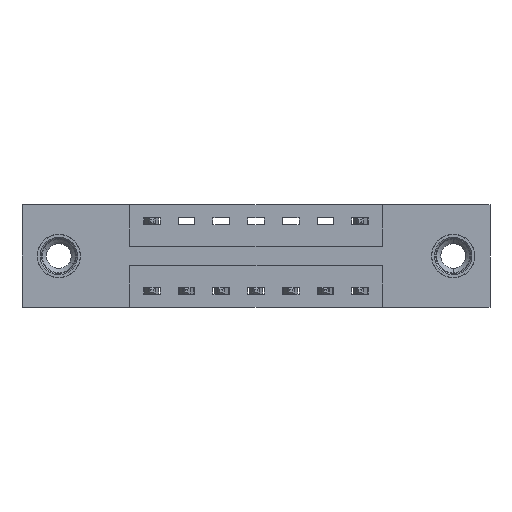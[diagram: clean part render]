
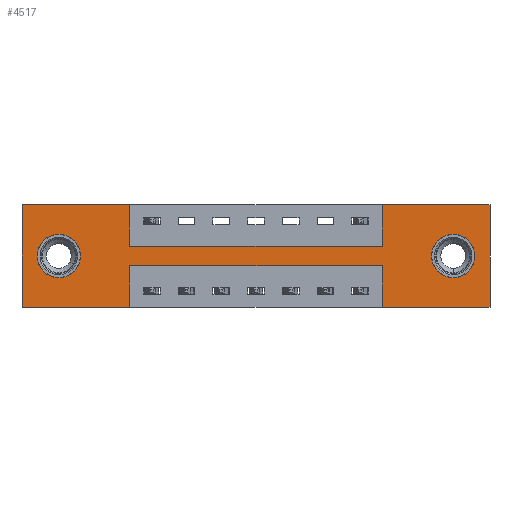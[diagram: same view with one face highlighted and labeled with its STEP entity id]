
A CAD part, front view. The second image highlights one B-rep face of the part: STEP entity #4517.
In plain terms, the highlighted planar face has unit normal (0, -1, 0).
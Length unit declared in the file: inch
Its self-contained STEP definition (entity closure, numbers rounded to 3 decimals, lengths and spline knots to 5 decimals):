
#27 = LINE ( 'NONE', #3414, #8600 ) ;
#93 = CARTESIAN_POINT ( 'NONE',  ( 1.2975, 0., -0.37 ) ) ;
#106 = CARTESIAN_POINT ( 'NONE',  ( 0.3875, 0., 0. ) ) ;
#147 = ORIENTED_EDGE ( 'NONE', *, *, #5257, .T. ) ;
#164 = VERTEX_POINT ( 'NONE', #93 ) ;
#167 = EDGE_CURVE ( 'NONE', #8975, #1400, #3425, .T. ) ;
#195 = CIRCLE ( 'NONE', #6165, 0.078 ) ;
#241 = CARTESIAN_POINT ( 'NONE',  ( 0.1325, 0., -0.263 ) ) ;
#291 = CARTESIAN_POINT ( 'NONE',  ( 0., 0., 0. ) ) ;
#565 = CARTESIAN_POINT ( 'NONE',  ( 0.1325, 0., -0.185 ) ) ;
#638 = CARTESIAN_POINT ( 'NONE',  ( 1.5525, 0., -0.263 ) ) ;
#639 = FACE_OUTER_BOUND ( 'NONE', #1988, .T. ) ;
#648 = AXIS2_PLACEMENT_3D ( 'NONE', #3900, #9489, #4722 ) ;
#661 = VECTOR ( 'NONE', #890, 39.37008 ) ;
#701 = CARTESIAN_POINT ( 'NONE',  ( 0., 0., -0.37 ) ) ;
#730 = VERTEX_POINT ( 'NONE', #6045 ) ;
#732 = EDGE_CURVE ( 'NONE', #3768, #1981, #9883, .T. ) ;
#786 = EDGE_CURVE ( 'NONE', #5219, #9329, #1160, .T. ) ;
#890 = DIRECTION ( 'NONE',  ( 0., 0., -1. ) ) ;
#899 = VECTOR ( 'NONE', #8381, 39.37008 ) ;
#1026 = DIRECTION ( 'NONE',  ( 0., 1., 0. ) ) ;
#1062 = ORIENTED_EDGE ( 'NONE', *, *, #4752, .F. ) ;
#1160 = LINE ( 'NONE', #1279, #899 ) ;
#1279 = CARTESIAN_POINT ( 'NONE',  ( 1.2975, 0., 0. ) ) ;
#1289 = LINE ( 'NONE', #8566, #7407 ) ;
#1358 = EDGE_CURVE ( 'NONE', #6492, #10025, #4766, .T. ) ;
#1366 = EDGE_LOOP ( 'NONE', ( #147, #7318 ) ) ;
#1400 = VERTEX_POINT ( 'NONE', #241 ) ;
#1449 = VERTEX_POINT ( 'NONE', #9149 ) ;
#1770 = VECTOR ( 'NONE', #5066, 39.37008 ) ;
#1893 = EDGE_CURVE ( 'NONE', #10025, #5219, #9355, .T. ) ;
#1908 = CIRCLE ( 'NONE', #6299, 0.078 ) ;
#1981 = VERTEX_POINT ( 'NONE', #8989 ) ;
#1988 = EDGE_LOOP ( 'NONE', ( #5203, #6474, #5142, #5419, #5060, #6479, #5100, #6022, #7809, #1062, #4306, #5007 ) ) ;
#2001 = VERTEX_POINT ( 'NONE', #7395 ) ;
#2034 = EDGE_CURVE ( 'NONE', #730, #3953, #27, .T. ) ;
#2105 = CARTESIAN_POINT ( 'NONE',  ( 0.3875, 0., -0.15 ) ) ;
#2164 = LINE ( 'NONE', #9965, #5908 ) ;
#2166 = LINE ( 'NONE', #7839, #4044 ) ;
#2369 = VECTOR ( 'NONE', #5772, 39.37008 ) ;
#2404 = VECTOR ( 'NONE', #4386, 39.37008 ) ;
#2504 = CARTESIAN_POINT ( 'NONE',  ( 0., 0., -0.37 ) ) ;
#2578 = CARTESIAN_POINT ( 'NONE',  ( 0., 0., 0. ) ) ;
#2607 = LINE ( 'NONE', #4992, #2369 ) ;
#2841 = DIRECTION ( 'NONE',  ( -1., 0., 0. ) ) ;
#3043 = CARTESIAN_POINT ( 'NONE',  ( 0.3875, 0., -0.22 ) ) ;
#3103 = DIRECTION ( 'NONE',  ( 0., 0., 1. ) ) ;
#3208 = VECTOR ( 'NONE', #8088, 39.37008 ) ;
#3414 = CARTESIAN_POINT ( 'NONE',  ( 1.685, 0., 0. ) ) ;
#3425 = CIRCLE ( 'NONE', #8593, 0.078 ) ;
#3467 = DIRECTION ( 'NONE',  ( 0., 1., 0. ) ) ;
#3490 = CARTESIAN_POINT ( 'NONE',  ( 0.1325, 0., -0.107 ) ) ;
#3691 = EDGE_CURVE ( 'NONE', #5584, #3768, #9450, .T. ) ;
#3768 = VERTEX_POINT ( 'NONE', #7400 ) ;
#3893 = LINE ( 'NONE', #2578, #1770 ) ;
#3900 = CARTESIAN_POINT ( 'NONE',  ( 0.1325, 0., -0.185 ) ) ;
#3953 = VERTEX_POINT ( 'NONE', #5197 ) ;
#4044 = VECTOR ( 'NONE', #8661, 39.37008 ) ;
#4130 = DIRECTION ( 'NONE',  ( 0., 0., -1. ) ) ;
#4132 = VERTEX_POINT ( 'NONE', #638 ) ;
#4243 = EDGE_CURVE ( 'NONE', #164, #8433, #1289, .T. ) ;
#4306 = ORIENTED_EDGE ( 'NONE', *, *, #5836, .F. ) ;
#4386 = DIRECTION ( 'NONE',  ( 1., 0., 0. ) ) ;
#4478 = CARTESIAN_POINT ( 'NONE',  ( 1.2975, 0., -0.22 ) ) ;
#4517 = ADVANCED_FACE ( 'NONE', ( #6817, #5187, #639 ), #8084, .T. ) ;
#4613 = DIRECTION ( 'NONE',  ( 0., 0., 1. ) ) ;
#4722 = DIRECTION ( 'NONE',  ( 0., 0., 1. ) ) ;
#4752 = EDGE_CURVE ( 'NONE', #1449, #6492, #4821, .T. ) ;
#4766 = LINE ( 'NONE', #5851, #10043 ) ;
#4798 = EDGE_CURVE ( 'NONE', #8433, #5584, #2164, .T. ) ;
#4821 = LINE ( 'NONE', #291, #2404 ) ;
#4992 = CARTESIAN_POINT ( 'NONE',  ( 0., 0., -0.37 ) ) ;
#5007 = ORIENTED_EDGE ( 'NONE', *, *, #732, .F. ) ;
#5060 = ORIENTED_EDGE ( 'NONE', *, *, #2034, .F. ) ;
#5063 = DIRECTION ( 'NONE',  ( 0., 0., -1. ) ) ;
#5066 = DIRECTION ( 'NONE',  ( 0., 0., 1. ) ) ;
#5100 = ORIENTED_EDGE ( 'NONE', *, *, #786, .F. ) ;
#5142 = ORIENTED_EDGE ( 'NONE', *, *, #4243, .F. ) ;
#5187 = FACE_BOUND ( 'NONE', #6036, .T. ) ;
#5197 = CARTESIAN_POINT ( 'NONE',  ( 1.685, 0., -0.37 ) ) ;
#5203 = ORIENTED_EDGE ( 'NONE', *, *, #3691, .F. ) ;
#5210 = CIRCLE ( 'NONE', #648, 0.078 ) ;
#5219 = VERTEX_POINT ( 'NONE', #9007 ) ;
#5257 = EDGE_CURVE ( 'NONE', #2001, #4132, #1908, .T. ) ;
#5419 = ORIENTED_EDGE ( 'NONE', *, *, #7109, .F. ) ;
#5584 = VERTEX_POINT ( 'NONE', #3043 ) ;
#5708 = CARTESIAN_POINT ( 'NONE',  ( 0.3875, 0., -0.37 ) ) ;
#5772 = DIRECTION ( 'NONE',  ( -1., 0., 0. ) ) ;
#5836 = EDGE_CURVE ( 'NONE', #1981, #1449, #3893, .T. ) ;
#5839 = CARTESIAN_POINT ( 'NONE',  ( 1.5525, 0., -0.185 ) ) ;
#5851 = CARTESIAN_POINT ( 'NONE',  ( 0.3875, 0., 0. ) ) ;
#5908 = VECTOR ( 'NONE', #2841, 39.37008 ) ;
#6022 = ORIENTED_EDGE ( 'NONE', *, *, #1893, .F. ) ;
#6036 = EDGE_LOOP ( 'NONE', ( #9484, #6417 ) ) ;
#6045 = CARTESIAN_POINT ( 'NONE',  ( 1.685, 0., 0. ) ) ;
#6165 = AXIS2_PLACEMENT_3D ( 'NONE', #5839, #1026, #6670 ) ;
#6299 = AXIS2_PLACEMENT_3D ( 'NONE', #8252, #3467, #9084 ) ;
#6417 = ORIENTED_EDGE ( 'NONE', *, *, #8698, .T. ) ;
#6474 = ORIENTED_EDGE ( 'NONE', *, *, #4798, .F. ) ;
#6479 = ORIENTED_EDGE ( 'NONE', *, *, #9879, .F. ) ;
#6492 = VERTEX_POINT ( 'NONE', #106 ) ;
#6670 = DIRECTION ( 'NONE',  ( 0., 0., -1. ) ) ;
#6817 = FACE_BOUND ( 'NONE', #1366, .T. ) ;
#7109 = EDGE_CURVE ( 'NONE', #3953, #164, #2607, .T. ) ;
#7126 = EDGE_CURVE ( 'NONE', #4132, #2001, #195, .T. ) ;
#7292 = CARTESIAN_POINT ( 'NONE',  ( 0.3875, 0., -0.15 ) ) ;
#7318 = ORIENTED_EDGE ( 'NONE', *, *, #7126, .T. ) ;
#7395 = CARTESIAN_POINT ( 'NONE',  ( 1.5525, 0., -0.107 ) ) ;
#7400 = CARTESIAN_POINT ( 'NONE',  ( 0.3875, 0., -0.37 ) ) ;
#7407 = VECTOR ( 'NONE', #4613, 39.37008 ) ;
#7792 = VECTOR ( 'NONE', #9769, 39.37008 ) ;
#7809 = ORIENTED_EDGE ( 'NONE', *, *, #1358, .F. ) ;
#7839 = CARTESIAN_POINT ( 'NONE',  ( 0., 0., 0. ) ) ;
#8084 = PLANE ( 'NONE',  #10026 ) ;
#8088 = DIRECTION ( 'NONE',  ( 1., 0., 0. ) ) ;
#8206 = DIRECTION ( 'NONE',  ( 0., 1., 0. ) ) ;
#8220 = DIRECTION ( 'NONE',  ( 0., 0., -1. ) ) ;
#8252 = CARTESIAN_POINT ( 'NONE',  ( 1.5525, 0., -0.185 ) ) ;
#8381 = DIRECTION ( 'NONE',  ( 0., 0., 1. ) ) ;
#8433 = VERTEX_POINT ( 'NONE', #4478 ) ;
#8566 = CARTESIAN_POINT ( 'NONE',  ( 1.2975, 0., -0.37 ) ) ;
#8593 = AXIS2_PLACEMENT_3D ( 'NONE', #565, #8206, #3103 ) ;
#8600 = VECTOR ( 'NONE', #5063, 39.37008 ) ;
#8661 = DIRECTION ( 'NONE',  ( 1., 0., 0. ) ) ;
#8698 = EDGE_CURVE ( 'NONE', #1400, #8975, #5210, .T. ) ;
#8912 = DIRECTION ( 'NONE',  ( 0., -1., 0. ) ) ;
#8975 = VERTEX_POINT ( 'NONE', #3490 ) ;
#8989 = CARTESIAN_POINT ( 'NONE',  ( 0., 0., -0.37 ) ) ;
#9007 = CARTESIAN_POINT ( 'NONE',  ( 1.2975, 0., -0.15 ) ) ;
#9084 = DIRECTION ( 'NONE',  ( 0., 0., -1. ) ) ;
#9149 = CARTESIAN_POINT ( 'NONE',  ( 0., 0., 0. ) ) ;
#9329 = VERTEX_POINT ( 'NONE', #10258 ) ;
#9355 = LINE ( 'NONE', #7292, #3208 ) ;
#9450 = LINE ( 'NONE', #5708, #661 ) ;
#9484 = ORIENTED_EDGE ( 'NONE', *, *, #167, .T. ) ;
#9489 = DIRECTION ( 'NONE',  ( 0., 1., 0. ) ) ;
#9769 = DIRECTION ( 'NONE',  ( -1., 0., 0. ) ) ;
#9879 = EDGE_CURVE ( 'NONE', #9329, #730, #2166, .T. ) ;
#9883 = LINE ( 'NONE', #701, #7792 ) ;
#9965 = CARTESIAN_POINT ( 'NONE',  ( 0.3875, 0., -0.22 ) ) ;
#10025 = VERTEX_POINT ( 'NONE', #2105 ) ;
#10026 = AXIS2_PLACEMENT_3D ( 'NONE', #2504, #8912, #4130 ) ;
#10043 = VECTOR ( 'NONE', #8220, 39.37008 ) ;
#10258 = CARTESIAN_POINT ( 'NONE',  ( 1.2975, 0., 0. ) ) ;
